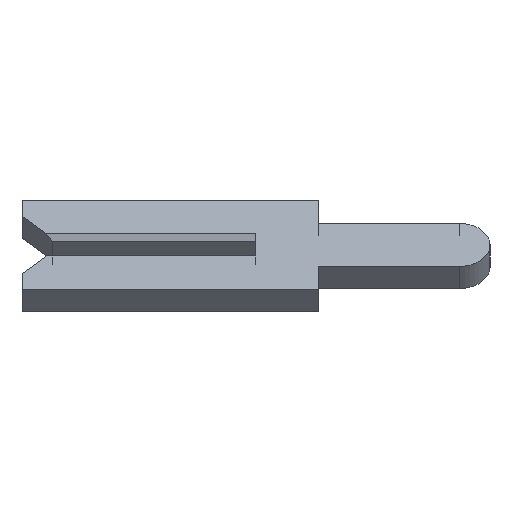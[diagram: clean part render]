
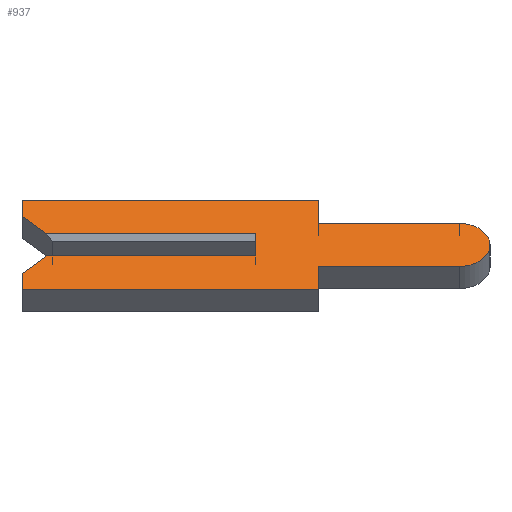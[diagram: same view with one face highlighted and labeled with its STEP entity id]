
A CAD part, left-side view. The second image highlights one B-rep face of the part: STEP entity #937.
In plain terms, the highlighted face is planar.
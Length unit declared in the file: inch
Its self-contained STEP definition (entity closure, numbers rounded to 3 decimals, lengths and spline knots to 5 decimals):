
#40 = VECTOR ( 'NONE', #1008, 39.37008 ) ;
#90 = VERTEX_POINT ( 'NONE', #644 ) ;
#103 = CARTESIAN_POINT ( 'NONE',  ( -0.01, 0.15, 0.026 ) ) ;
#111 = ORIENTED_EDGE ( 'NONE', *, *, #1325, .F. ) ;
#130 = EDGE_CURVE ( 'NONE', #862, #1092, #886, .T. ) ;
#140 = VECTOR ( 'NONE', #359, 39.37008 ) ;
#161 = CARTESIAN_POINT ( 'NONE',  ( -0.01, 0.15, 0.04 ) ) ;
#170 = VERTEX_POINT ( 'NONE', #440 ) ;
#178 = EDGE_CURVE ( 'NONE', #1239, #484, #1356, .T. ) ;
#206 = EDGE_CURVE ( 'NONE', #1256, #1174, #851, .T. ) ;
#207 = VECTOR ( 'NONE', #571, 39.37008 ) ;
#214 = EDGE_CURVE ( 'NONE', #1203, #90, #245, .T. ) ;
#217 = DIRECTION ( 'NONE',  ( 0., 0., -1. ) ) ;
#222 = AXIS2_PLACEMENT_3D ( 'NONE', #327, #563, #217 ) ;
#229 = CARTESIAN_POINT ( 'NONE',  ( -0.01, 0.1305, -0.0065 ) ) ;
#237 = CARTESIAN_POINT ( 'NONE',  ( -0.01, -0.1305, 0.0195 ) ) ;
#245 = LINE ( 'NONE', #1125, #1135 ) ;
#246 = CARTESIAN_POINT ( 'NONE',  ( -0.01, 0.15, -0.04 ) ) ;
#249 = CARTESIAN_POINT ( 'NONE',  ( -0.01, 0.15, -0.026 ) ) ;
#262 = VECTOR ( 'NONE', #445, 39.37008 ) ;
#266 = EDGE_CURVE ( 'NONE', #576, #170, #1094, .T. ) ;
#282 = LINE ( 'NONE', #825, #748 ) ;
#289 = EDGE_CURVE ( 'NONE', #757, #1367, #907, .T. ) ;
#290 = VECTOR ( 'NONE', #660, 39.37008 ) ;
#304 = VERTEX_POINT ( 'NONE', #841 ) ;
#308 = AXIS2_PLACEMENT_3D ( 'NONE', #1259, #936, #1148 ) ;
#327 = CARTESIAN_POINT ( 'NONE',  ( -0.01, -0.1305, 0. ) ) ;
#332 = CARTESIAN_POINT ( 'NONE',  ( -0.01, 0., 0.01 ) ) ;
#359 = DIRECTION ( 'NONE',  ( 0., 0., 1. ) ) ;
#364 = EDGE_CURVE ( 'NONE', #304, #1203, #596, .T. ) ;
#370 = ORIENTED_EDGE ( 'NONE', *, *, #827, .F. ) ;
#373 = ORIENTED_EDGE ( 'NONE', *, *, #1146, .F. ) ;
#379 = LINE ( 'NONE', #393, #1299 ) ;
#384 = LINE ( 'NONE', #1249, #262 ) ;
#393 = CARTESIAN_POINT ( 'NONE',  ( -0.01, -0.1305, -0.01 ) ) ;
#410 = EDGE_CURVE ( 'NONE', #484, #862, #379, .T. ) ;
#425 = EDGE_CURVE ( 'NONE', #1256, #1092, #1159, .T. ) ;
#440 = CARTESIAN_POINT ( 'NONE',  ( -0.01, -0.04, 0.04 ) ) ;
#445 = DIRECTION ( 'NONE',  ( 0., 1., 0. ) ) ;
#463 = CARTESIAN_POINT ( 'NONE',  ( -0.01, 0.15, -0.026 ) ) ;
#479 = ORIENTED_EDGE ( 'NONE', *, *, #425, .T. ) ;
#484 = VERTEX_POINT ( 'NONE', #496 ) ;
#496 = CARTESIAN_POINT ( 'NONE',  ( -0.01, 0.134, -0.01 ) ) ;
#519 = ORIENTED_EDGE ( 'NONE', *, *, #214, .F. ) ;
#531 = VERTEX_POINT ( 'NONE', #246 ) ;
#540 = VECTOR ( 'NONE', #1466, 39.37008 ) ;
#560 = CARTESIAN_POINT ( 'NONE',  ( -0.01, 0.15, 0.04 ) ) ;
#563 = DIRECTION ( 'NONE',  ( 1., 0., 0. ) ) ;
#571 = DIRECTION ( 'NONE',  ( 0., -1., 0. ) ) ;
#576 = VERTEX_POINT ( 'NONE', #161 ) ;
#596 = LINE ( 'NONE', #929, #1169 ) ;
#610 = CARTESIAN_POINT ( 'NONE',  ( -0.01, 0.15, 0.01 ) ) ;
#644 = CARTESIAN_POINT ( 'NONE',  ( -0.01, -0.04, -0.04 ) ) ;
#660 = DIRECTION ( 'NONE',  ( 0., -1., 0. ) ) ;
#683 = CARTESIAN_POINT ( 'NONE',  ( -0.01, 0., -0.01 ) ) ;
#707 = DIRECTION ( 'NONE',  ( 0., 0., -1. ) ) ;
#748 = VECTOR ( 'NONE', #707, 39.37008 ) ;
#757 = VERTEX_POINT ( 'NONE', #1426 ) ;
#786 = DIRECTION ( 'NONE',  ( 0., 0., -1. ) ) ;
#799 = CARTESIAN_POINT ( 'NONE',  ( -0.01, -0.04, 0.0195 ) ) ;
#804 = VECTOR ( 'NONE', #1368, 39.37008 ) ;
#822 = DIRECTION ( 'NONE',  ( 0., -1., 0. ) ) ;
#825 = CARTESIAN_POINT ( 'NONE',  ( -0.01, -0.04, 0.04 ) ) ;
#827 = EDGE_CURVE ( 'NONE', #1174, #576, #1233, .T. ) ;
#841 = CARTESIAN_POINT ( 'NONE',  ( -0.01, -0.1305, -0.0195 ) ) ;
#851 = LINE ( 'NONE', #1119, #540 ) ;
#862 = VERTEX_POINT ( 'NONE', #683 ) ;
#875 = FACE_OUTER_BOUND ( 'NONE', #1124, .T. ) ;
#883 = ORIENTED_EDGE ( 'NONE', *, *, #1204, .F. ) ;
#886 = LINE ( 'NONE', #1013, #1114 ) ;
#899 = DIRECTION ( 'NONE',  ( 0., 0., 1. ) ) ;
#907 = LINE ( 'NONE', #799, #290 ) ;
#915 = ORIENTED_EDGE ( 'NONE', *, *, #364, .F. ) ;
#929 = CARTESIAN_POINT ( 'NONE',  ( -0.01, -0.04, -0.0195 ) ) ;
#934 = VECTOR ( 'NONE', #1461, 39.37008 ) ;
#936 = DIRECTION ( 'NONE',  ( 1., 0., 0. ) ) ;
#937 = ADVANCED_FACE ( 'NONE', ( #875 ), #1243, .F. ) ;
#948 = EDGE_CURVE ( 'NONE', #90, #531, #384, .T. ) ;
#1008 = DIRECTION ( 'NONE',  ( 0., -0.707, 0.707 ) ) ;
#1013 = CARTESIAN_POINT ( 'NONE',  ( -0.01, 0., 0.0065 ) ) ;
#1039 = DIRECTION ( 'NONE',  ( 0., 1., 0. ) ) ;
#1056 = ORIENTED_EDGE ( 'NONE', *, *, #130, .F. ) ;
#1092 = VERTEX_POINT ( 'NONE', #332 ) ;
#1094 = LINE ( 'NONE', #560, #804 ) ;
#1114 = VECTOR ( 'NONE', #899, 39.37008 ) ;
#1119 = CARTESIAN_POINT ( 'NONE',  ( -0.01, 0.1305, 0.0065 ) ) ;
#1124 = EDGE_LOOP ( 'NONE', ( #479, #1056, #1152, #1208, #111, #1129, #519, #915, #373, #1147, #883, #1354, #370, #1326 ) ) ;
#1125 = CARTESIAN_POINT ( 'NONE',  ( -0.01, -0.04, -0.04 ) ) ;
#1129 = ORIENTED_EDGE ( 'NONE', *, *, #948, .F. ) ;
#1135 = VECTOR ( 'NONE', #786, 39.37008 ) ;
#1146 = EDGE_CURVE ( 'NONE', #1367, #304, #1197, .T. ) ;
#1147 = ORIENTED_EDGE ( 'NONE', *, *, #289, .F. ) ;
#1148 = DIRECTION ( 'NONE',  ( 0., 0., -1. ) ) ;
#1152 = ORIENTED_EDGE ( 'NONE', *, *, #410, .F. ) ;
#1159 = LINE ( 'NONE', #610, #207 ) ;
#1164 = CARTESIAN_POINT ( 'NONE',  ( -0.01, 0.134, 0.01 ) ) ;
#1169 = VECTOR ( 'NONE', #1039, 39.37008 ) ;
#1174 = VERTEX_POINT ( 'NONE', #1388 ) ;
#1197 = CIRCLE ( 'NONE', #308, 0.0195 ) ;
#1203 = VERTEX_POINT ( 'NONE', #1275 ) ;
#1204 = EDGE_CURVE ( 'NONE', #170, #757, #282, .T. ) ;
#1208 = ORIENTED_EDGE ( 'NONE', *, *, #178, .F. ) ;
#1233 = LINE ( 'NONE', #103, #934 ) ;
#1239 = VERTEX_POINT ( 'NONE', #249 ) ;
#1243 = PLANE ( 'NONE',  #222 ) ;
#1249 = CARTESIAN_POINT ( 'NONE',  ( -0.01, 0.15, -0.04 ) ) ;
#1256 = VERTEX_POINT ( 'NONE', #1164 ) ;
#1259 = CARTESIAN_POINT ( 'NONE',  ( -0.01, -0.1305, 0. ) ) ;
#1275 = CARTESIAN_POINT ( 'NONE',  ( -0.01, -0.04, -0.0195 ) ) ;
#1299 = VECTOR ( 'NONE', #822, 39.37008 ) ;
#1325 = EDGE_CURVE ( 'NONE', #531, #1239, #1430, .T. ) ;
#1326 = ORIENTED_EDGE ( 'NONE', *, *, #206, .F. ) ;
#1354 = ORIENTED_EDGE ( 'NONE', *, *, #266, .F. ) ;
#1356 = LINE ( 'NONE', #229, #40 ) ;
#1367 = VERTEX_POINT ( 'NONE', #237 ) ;
#1368 = DIRECTION ( 'NONE',  ( 0., -1., 0. ) ) ;
#1388 = CARTESIAN_POINT ( 'NONE',  ( -0.01, 0.15, 0.026 ) ) ;
#1426 = CARTESIAN_POINT ( 'NONE',  ( -0.01, -0.04, 0.0195 ) ) ;
#1430 = LINE ( 'NONE', #463, #140 ) ;
#1461 = DIRECTION ( 'NONE',  ( 0., 0., 1. ) ) ;
#1466 = DIRECTION ( 'NONE',  ( 0., 0.707, 0.707 ) ) ;
